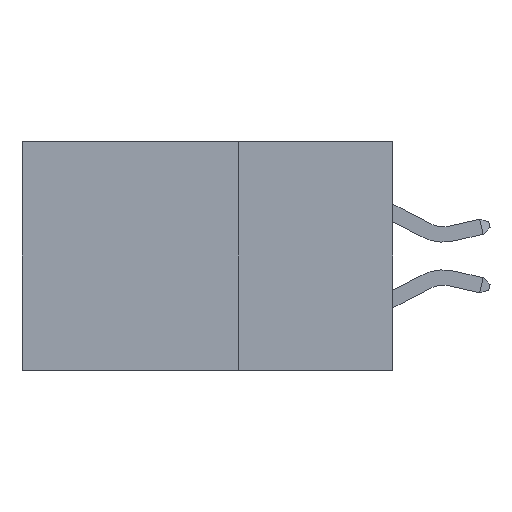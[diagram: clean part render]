
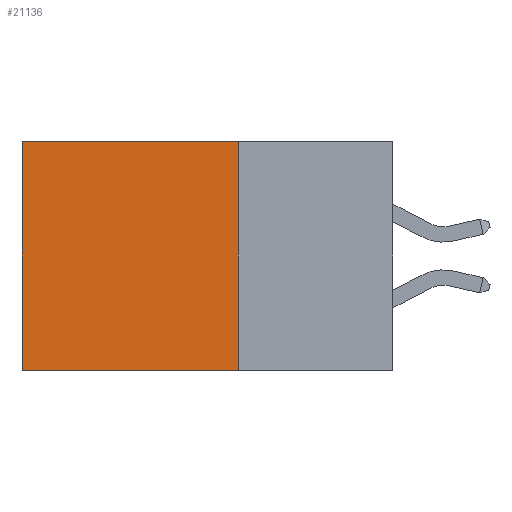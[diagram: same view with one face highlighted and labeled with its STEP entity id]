
A CAD part, left-side view. The second image highlights one B-rep face of the part: STEP entity #21136.
In plain terms, the highlighted planar face has unit normal (-1, 0, 0).
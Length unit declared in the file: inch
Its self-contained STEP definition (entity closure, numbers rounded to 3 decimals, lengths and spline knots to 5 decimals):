
#155 = CARTESIAN_POINT ( 'NONE',  ( 0.2875, 0.6, 0. ) ) ;
#330 = AXIS2_PLACEMENT_3D ( 'NONE', #8107, #35286, #29187 ) ;
#567 = VERTEX_POINT ( 'NONE', #24471 ) ;
#1723 = VECTOR ( 'NONE', #9680, 39.37008 ) ;
#5745 = EDGE_LOOP ( 'NONE', ( #24621, #10929, #17228, #38167 ) ) ;
#6508 = LINE ( 'NONE', #33267, #23484 ) ;
#6724 = LINE ( 'NONE', #7113, #30304 ) ;
#7113 = CARTESIAN_POINT ( 'NONE',  ( 0.2875, 0.6, 0. ) ) ;
#8107 = CARTESIAN_POINT ( 'NONE',  ( 0.2875, 0.25, 0. ) ) ;
#9680 = DIRECTION ( 'NONE',  ( 0., 1., 0. ) ) ;
#10929 = ORIENTED_EDGE ( 'NONE', *, *, #28670, .F. ) ;
#13603 = CARTESIAN_POINT ( 'NONE',  ( 0.2875, 0.25, -0.37 ) ) ;
#14004 = PLANE ( 'NONE',  #330 ) ;
#14313 = CARTESIAN_POINT ( 'NONE',  ( 0.2875, 0.25, 0. ) ) ;
#15094 = DIRECTION ( 'NONE',  ( 0., 0., -1. ) ) ;
#16985 = VERTEX_POINT ( 'NONE', #13603 ) ;
#17228 = ORIENTED_EDGE ( 'NONE', *, *, #24901, .F. ) ;
#18252 = CARTESIAN_POINT ( 'NONE',  ( 0.2875, 0.25, -0.37 ) ) ;
#19277 = CARTESIAN_POINT ( 'NONE',  ( 0.2875, 0.25, 0. ) ) ;
#19870 = FACE_OUTER_BOUND ( 'NONE', #5745, .T. ) ;
#20001 = VERTEX_POINT ( 'NONE', #155 ) ;
#20582 = LINE ( 'NONE', #18252, #1723 ) ;
#21136 = ADVANCED_FACE ( 'NONE', ( #19870 ), #14004, .F. ) ;
#22517 = EDGE_CURVE ( 'NONE', #34577, #20001, #6508, .T. ) ;
#23484 = VECTOR ( 'NONE', #33533, 39.37008 ) ;
#24471 = CARTESIAN_POINT ( 'NONE',  ( 0.2875, 0.6, -0.37 ) ) ;
#24621 = ORIENTED_EDGE ( 'NONE', *, *, #35092, .T. ) ;
#24901 = EDGE_CURVE ( 'NONE', #34577, #16985, #29955, .T. ) ;
#25685 = VECTOR ( 'NONE', #15094, 39.37008 ) ;
#28670 = EDGE_CURVE ( 'NONE', #16985, #567, #20582, .T. ) ;
#29187 = DIRECTION ( 'NONE',  ( 0., 0., -1. ) ) ;
#29955 = LINE ( 'NONE', #14313, #25685 ) ;
#30304 = VECTOR ( 'NONE', #34286, 39.37008 ) ;
#33267 = CARTESIAN_POINT ( 'NONE',  ( 0.2875, 0.25, 0. ) ) ;
#33533 = DIRECTION ( 'NONE',  ( 0., 1., 0. ) ) ;
#34286 = DIRECTION ( 'NONE',  ( 0., 0., -1. ) ) ;
#34577 = VERTEX_POINT ( 'NONE', #19277 ) ;
#35092 = EDGE_CURVE ( 'NONE', #20001, #567, #6724, .T. ) ;
#35286 = DIRECTION ( 'NONE',  ( 1., 0., 0. ) ) ;
#38167 = ORIENTED_EDGE ( 'NONE', *, *, #22517, .T. ) ;
